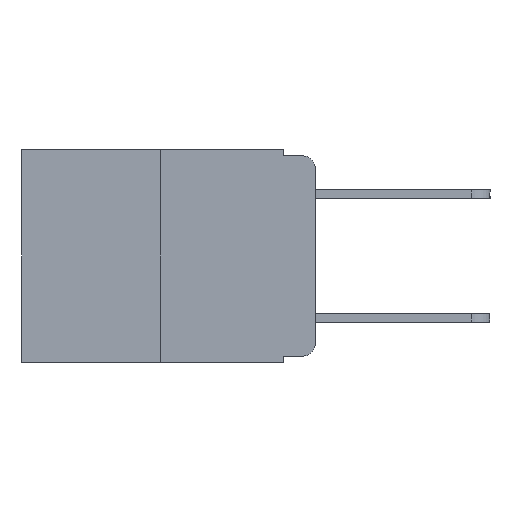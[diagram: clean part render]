
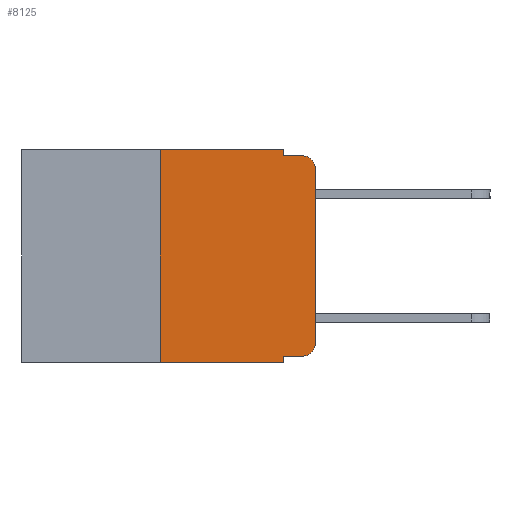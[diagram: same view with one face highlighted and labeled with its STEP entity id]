
A CAD part, left-side view. The second image highlights one B-rep face of the part: STEP entity #8125.
In plain terms, the highlighted planar face has unit normal (-1, 0, 0).
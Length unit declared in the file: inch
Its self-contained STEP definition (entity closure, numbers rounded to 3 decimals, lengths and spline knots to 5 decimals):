
#66 = DIRECTION ( 'NONE',  ( -1., 0., 0. ) ) ;
#551 = LINE ( 'NONE', #4797, #12866 ) ;
#791 = CARTESIAN_POINT ( 'NONE',  ( 0., 0.25, 0. ) ) ;
#1354 = VERTEX_POINT ( 'NONE', #11029 ) ;
#1418 = CARTESIAN_POINT ( 'NONE',  ( 0., 0.051, -0.343 ) ) ;
#1635 = ORIENTED_EDGE ( 'NONE', *, *, #1700, .F. ) ;
#1657 = ORIENTED_EDGE ( 'NONE', *, *, #3482, .F. ) ;
#1670 = PLANE ( 'NONE',  #9081 ) ;
#1700 = EDGE_CURVE ( 'NONE', #8376, #1354, #551, .T. ) ;
#1782 = FACE_OUTER_BOUND ( 'NONE', #2665, .T. ) ;
#2001 = DIRECTION ( 'NONE',  ( 0., 0., -1. ) ) ;
#2196 = CARTESIAN_POINT ( 'NONE',  ( 0., 0.473, -0.343 ) ) ;
#2242 = ORIENTED_EDGE ( 'NONE', *, *, #3459, .T. ) ;
#2323 = VECTOR ( 'NONE', #7803, 39.37008 ) ;
#2495 = ORIENTED_EDGE ( 'NONE', *, *, #3532, .F. ) ;
#2620 = ORIENTED_EDGE ( 'NONE', *, *, #3453, .T. ) ;
#2662 = ORIENTED_EDGE ( 'NONE', *, *, #3752, .F. ) ;
#2665 = EDGE_LOOP ( 'NONE', ( #2620, #2242, #1657, #2495, #1635, #6516, #7048, #2662, #4897, #4955 ) ) ;
#2683 = LINE ( 'NONE', #8606, #5614 ) ;
#2901 = EDGE_CURVE ( 'NONE', #4930, #3157, #2911, .T. ) ;
#2911 = LINE ( 'NONE', #2196, #8775 ) ;
#2915 = CARTESIAN_POINT ( 'NONE',  ( 0., 0.473, 0. ) ) ;
#3157 = VERTEX_POINT ( 'NONE', #1418 ) ;
#3212 = VERTEX_POINT ( 'NONE', #6102 ) ;
#3373 = VERTEX_POINT ( 'NONE', #9622 ) ;
#3378 = DIRECTION ( 'NONE',  ( 0., -1., 0. ) ) ;
#3453 = EDGE_CURVE ( 'NONE', #3212, #11355, #5628, .T. ) ;
#3459 = EDGE_CURVE ( 'NONE', #11355, #9974, #5272, .T. ) ;
#3463 = LINE ( 'NONE', #9365, #5990 ) ;
#3482 = EDGE_CURVE ( 'NONE', #5044, #9974, #7906, .T. ) ;
#3532 = EDGE_CURVE ( 'NONE', #1354, #5044, #7229, .T. ) ;
#3725 = EDGE_CURVE ( 'NONE', #4930, #8376, #11904, .T. ) ;
#3752 = EDGE_CURVE ( 'NONE', #3373, #3157, #3463, .T. ) ;
#3774 = EDGE_CURVE ( 'NONE', #3373, #10605, #2683, .T. ) ;
#3800 = EDGE_CURVE ( 'NONE', #10605, #3212, #8540, .T. ) ;
#4094 = VECTOR ( 'NONE', #12571, 39.37008 ) ;
#4747 = DIRECTION ( 'NONE',  ( 0., -1., 0. ) ) ;
#4797 = CARTESIAN_POINT ( 'NONE',  ( 0., 0.473, 0. ) ) ;
#4897 = ORIENTED_EDGE ( 'NONE', *, *, #3774, .T. ) ;
#4930 = VERTEX_POINT ( 'NONE', #8031 ) ;
#4955 = ORIENTED_EDGE ( 'NONE', *, *, #3800, .T. ) ;
#5044 = VERTEX_POINT ( 'NONE', #7179 ) ;
#5176 = CARTESIAN_POINT ( 'NONE',  ( 0., 0.02, -0.01 ) ) ;
#5272 = CIRCLE ( 'NONE', #9833, 0.02 ) ;
#5614 = VECTOR ( 'NONE', #6036, 39.37008 ) ;
#5628 = LINE ( 'NONE', #7828, #2323 ) ;
#5990 = VECTOR ( 'NONE', #8203, 39.37008 ) ;
#6036 = DIRECTION ( 'NONE',  ( 0., -1., 0. ) ) ;
#6102 = CARTESIAN_POINT ( 'NONE',  ( 0., 0., -0.313 ) ) ;
#6516 = ORIENTED_EDGE ( 'NONE', *, *, #3725, .F. ) ;
#6625 = DIRECTION ( 'NONE',  ( 1., 0., 0. ) ) ;
#7048 = ORIENTED_EDGE ( 'NONE', *, *, #2901, .T. ) ;
#7179 = CARTESIAN_POINT ( 'NONE',  ( 0., 0.051, -0.01 ) ) ;
#7229 = LINE ( 'NONE', #12586, #4094 ) ;
#7803 = DIRECTION ( 'NONE',  ( 0., 0., 1. ) ) ;
#7828 = CARTESIAN_POINT ( 'NONE',  ( 0., 0., 0. ) ) ;
#7906 = LINE ( 'NONE', #13226, #10632 ) ;
#8031 = CARTESIAN_POINT ( 'NONE',  ( 0., 0.25, -0.343 ) ) ;
#8125 = ADVANCED_FACE ( 'NONE', ( #1782 ), #1670, .F. ) ;
#8203 = DIRECTION ( 'NONE',  ( 0., 0., -1. ) ) ;
#8245 = CARTESIAN_POINT ( 'NONE',  ( 0., 0.25, 0. ) ) ;
#8376 = VERTEX_POINT ( 'NONE', #791 ) ;
#8540 = CIRCLE ( 'NONE', #11110, 0.02 ) ;
#8606 = CARTESIAN_POINT ( 'NONE',  ( 0., 0.051, -0.333 ) ) ;
#8688 = CARTESIAN_POINT ( 'NONE',  ( 0., 0.02, -0.313 ) ) ;
#8775 = VECTOR ( 'NONE', #3378, 39.37008 ) ;
#9081 = AXIS2_PLACEMENT_3D ( 'NONE', #2915, #6625, #13699 ) ;
#9365 = CARTESIAN_POINT ( 'NONE',  ( 0., 0.051, 0. ) ) ;
#9523 = VECTOR ( 'NONE', #11074, 39.37008 ) ;
#9622 = CARTESIAN_POINT ( 'NONE',  ( 0., 0.051, -0.333 ) ) ;
#9833 = AXIS2_PLACEMENT_3D ( 'NONE', #10896, #10881, #10666 ) ;
#9974 = VERTEX_POINT ( 'NONE', #5176 ) ;
#10605 = VERTEX_POINT ( 'NONE', #12943 ) ;
#10632 = VECTOR ( 'NONE', #13191, 39.37008 ) ;
#10666 = DIRECTION ( 'NONE',  ( 0., 0., -1. ) ) ;
#10881 = DIRECTION ( 'NONE',  ( -1., 0., 0. ) ) ;
#10896 = CARTESIAN_POINT ( 'NONE',  ( 0., 0.02, -0.03 ) ) ;
#11029 = CARTESIAN_POINT ( 'NONE',  ( 0., 0.051, 0. ) ) ;
#11074 = DIRECTION ( 'NONE',  ( 0., 0., 1. ) ) ;
#11110 = AXIS2_PLACEMENT_3D ( 'NONE', #8688, #66, #2001 ) ;
#11355 = VERTEX_POINT ( 'NONE', #12966 ) ;
#11904 = LINE ( 'NONE', #8245, #9523 ) ;
#12571 = DIRECTION ( 'NONE',  ( 0., 0., -1. ) ) ;
#12586 = CARTESIAN_POINT ( 'NONE',  ( 0., 0.051, 0. ) ) ;
#12866 = VECTOR ( 'NONE', #4747, 39.37008 ) ;
#12943 = CARTESIAN_POINT ( 'NONE',  ( 0., 0.02, -0.333 ) ) ;
#12966 = CARTESIAN_POINT ( 'NONE',  ( 0., 0., -0.03 ) ) ;
#13191 = DIRECTION ( 'NONE',  ( 0., -1., 0. ) ) ;
#13226 = CARTESIAN_POINT ( 'NONE',  ( 0., 0.051, -0.01 ) ) ;
#13699 = DIRECTION ( 'NONE',  ( 0., 0., -1. ) ) ;
